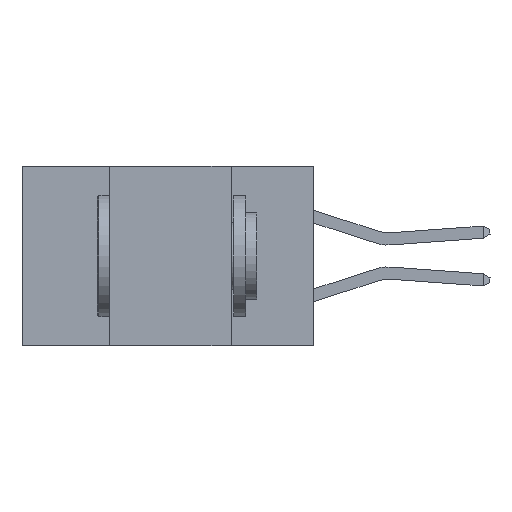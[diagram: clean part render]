
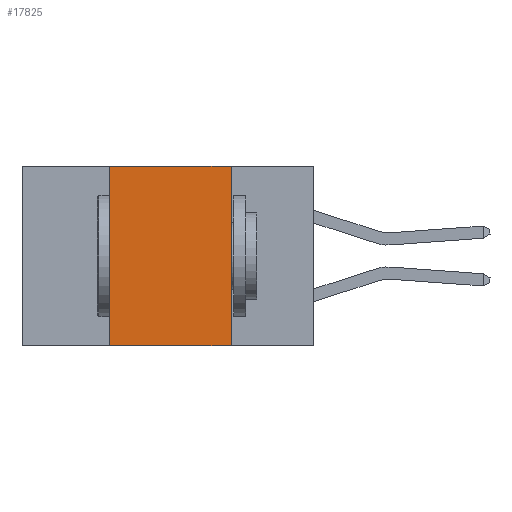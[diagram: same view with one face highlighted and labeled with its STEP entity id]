
A CAD part, left-side view. The second image highlights one B-rep face of the part: STEP entity #17825.
In plain terms, the highlighted planar face has unit normal (-1, 0, 0).
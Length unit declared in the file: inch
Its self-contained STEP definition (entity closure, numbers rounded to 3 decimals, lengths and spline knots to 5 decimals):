
#1172 = LINE ( 'NONE', #1410, #24787 ) ;
#1410 = CARTESIAN_POINT ( 'NONE',  ( 0., 0.42, 0. ) ) ;
#1977 = VERTEX_POINT ( 'NONE', #35921 ) ;
#6000 = LINE ( 'NONE', #17283, #38187 ) ;
#8102 = VECTOR ( 'NONE', #33902, 39.37008 ) ;
#8160 = VERTEX_POINT ( 'NONE', #26310 ) ;
#8701 = DIRECTION ( 'NONE',  ( 0., -1., 0. ) ) ;
#9375 = CARTESIAN_POINT ( 'NONE',  ( 0., 0.6, 0. ) ) ;
#10135 = FACE_OUTER_BOUND ( 'NONE', #28347, .T. ) ;
#11397 = CARTESIAN_POINT ( 'NONE',  ( 0., 0.6, -0.37 ) ) ;
#13631 = DIRECTION ( 'NONE',  ( 0., 0., -1. ) ) ;
#15536 = ORIENTED_EDGE ( 'NONE', *, *, #17908, .T. ) ;
#16694 = CARTESIAN_POINT ( 'NONE',  ( 0., 0.42, -0.37 ) ) ;
#16882 = AXIS2_PLACEMENT_3D ( 'NONE', #9375, #35095, #22901 ) ;
#17066 = EDGE_CURVE ( 'NONE', #39529, #25628, #1172, .T. ) ;
#17283 = CARTESIAN_POINT ( 'NONE',  ( 0., 0.17, 0. ) ) ;
#17579 = DIRECTION ( 'NONE',  ( 0., 0., 1. ) ) ;
#17825 = ADVANCED_FACE ( 'NONE', ( #10135 ), #22183, .F. ) ;
#17908 = EDGE_CURVE ( 'NONE', #39529, #1977, #30321, .T. ) ;
#22183 = PLANE ( 'NONE',  #16882 ) ;
#22901 = DIRECTION ( 'NONE',  ( 0., 0., -1. ) ) ;
#24452 = EDGE_CURVE ( 'NONE', #8160, #1977, #6000, .T. ) ;
#24787 = VECTOR ( 'NONE', #17579, 39.37008 ) ;
#25628 = VERTEX_POINT ( 'NONE', #28066 ) ;
#26310 = CARTESIAN_POINT ( 'NONE',  ( 0., 0.17, 0. ) ) ;
#27999 = CARTESIAN_POINT ( 'NONE',  ( 0., 0.6, 0. ) ) ;
#28066 = CARTESIAN_POINT ( 'NONE',  ( 0., 0.42, 0. ) ) ;
#28273 = VECTOR ( 'NONE', #8701, 39.37008 ) ;
#28347 = EDGE_LOOP ( 'NONE', ( #35934, #37898, #40838, #15536 ) ) ;
#29289 = LINE ( 'NONE', #27999, #28273 ) ;
#30321 = LINE ( 'NONE', #11397, #8102 ) ;
#31266 = EDGE_CURVE ( 'NONE', #25628, #8160, #29289, .T. ) ;
#33902 = DIRECTION ( 'NONE',  ( 0., -1., 0. ) ) ;
#35095 = DIRECTION ( 'NONE',  ( 1., 0., 0. ) ) ;
#35921 = CARTESIAN_POINT ( 'NONE',  ( 0., 0.17, -0.37 ) ) ;
#35934 = ORIENTED_EDGE ( 'NONE', *, *, #24452, .F. ) ;
#37898 = ORIENTED_EDGE ( 'NONE', *, *, #31266, .F. ) ;
#38187 = VECTOR ( 'NONE', #13631, 39.37008 ) ;
#39529 = VERTEX_POINT ( 'NONE', #16694 ) ;
#40838 = ORIENTED_EDGE ( 'NONE', *, *, #17066, .F. ) ;
